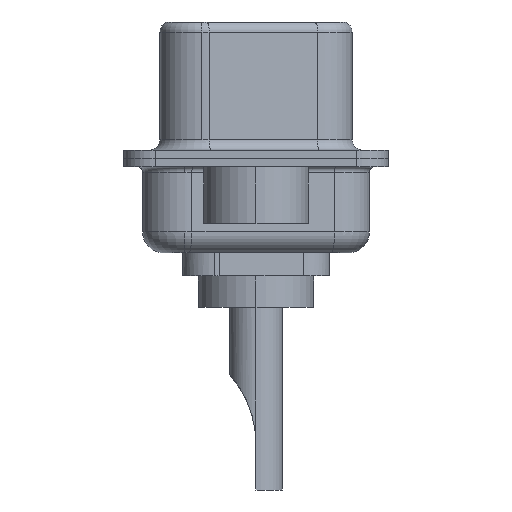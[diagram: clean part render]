
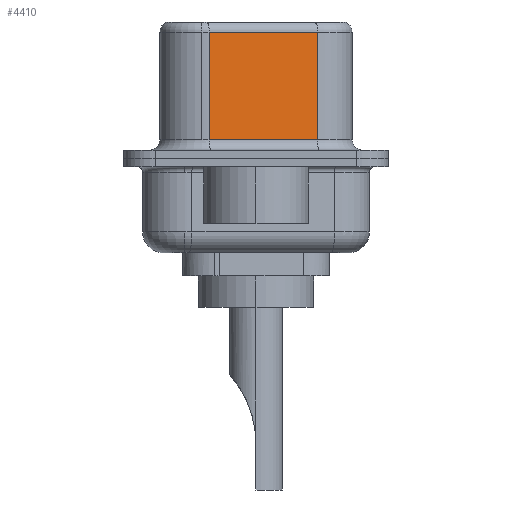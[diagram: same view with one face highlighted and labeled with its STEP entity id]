
A CAD part, left-side view. The second image highlights one B-rep face of the part: STEP entity #4410.
In plain terms, the highlighted planar face has unit normal (-0.985, -0.174, 0).
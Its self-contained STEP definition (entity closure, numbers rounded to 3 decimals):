
#92 = CARTESIAN_POINT ( 'NONE',  ( 4.585, -2.927, 6.52 ) ) ;
#216 = DIRECTION ( 'NONE',  ( 0., 0., -1. ) ) ;
#671 = VERTEX_POINT ( 'NONE', #15368 ) ;
#1027 = VERTEX_POINT ( 'NONE', #1853 ) ;
#1247 = VECTOR ( 'NONE', #216, 1000. ) ;
#1521 = DIRECTION ( 'NONE',  ( 0.174, -0.985, 0. ) ) ;
#1773 = EDGE_CURVE ( 'NONE', #671, #15665, #8259, .T. ) ;
#1853 = CARTESIAN_POINT ( 'NONE',  ( 3.675, 2.233, 6.02 ) ) ;
#1908 = FACE_OUTER_BOUND ( 'NONE', #16865, .T. ) ;
#1952 = VECTOR ( 'NONE', #1521, 1000. ) ;
#3297 = EDGE_CURVE ( 'NONE', #3618, #15665, #16054, .T. ) ;
#3618 = VERTEX_POINT ( 'NONE', #10603 ) ;
#3769 = ORIENTED_EDGE ( 'NONE', *, *, #8292, .T. ) ;
#4311 = CARTESIAN_POINT ( 'NONE',  ( 4.585, -2.927, 6.02 ) ) ;
#4410 = ADVANCED_FACE ( 'NONE', ( #1908 ), #14318, .F. ) ;
#6431 = VECTOR ( 'NONE', #6454, 1000. ) ;
#6454 = DIRECTION ( 'NONE',  ( 0., 0., -1. ) ) ;
#6577 = DIRECTION ( 'NONE',  ( -0.174, 0.985, 0. ) ) ;
#6581 = DIRECTION ( 'NONE',  ( 0.985, 0.174, 0. ) ) ;
#8259 = LINE ( 'NONE', #92, #1247 ) ;
#8292 = EDGE_CURVE ( 'NONE', #1027, #3618, #9884, .T. ) ;
#8526 = VECTOR ( 'NONE', #12195, 1000. ) ;
#9026 = CARTESIAN_POINT ( 'NONE',  ( 3.675, 2.233, 6.52 ) ) ;
#9884 = LINE ( 'NONE', #9026, #6431 ) ;
#10603 = CARTESIAN_POINT ( 'NONE',  ( 3.675, 2.233, 0.9 ) ) ;
#11206 = AXIS2_PLACEMENT_3D ( 'NONE', #13846, #6581, #6577 ) ;
#11610 = ORIENTED_EDGE ( 'NONE', *, *, #1773, .F. ) ;
#11935 = CARTESIAN_POINT ( 'NONE',  ( 4.585, -2.927, 0.9 ) ) ;
#12065 = EDGE_CURVE ( 'NONE', #671, #1027, #15632, .T. ) ;
#12195 = DIRECTION ( 'NONE',  ( -0.174, 0.985, 0. ) ) ;
#13846 = CARTESIAN_POINT ( 'NONE',  ( 4.585, -2.927, 6.52 ) ) ;
#14318 = PLANE ( 'NONE',  #11206 ) ;
#14711 = ORIENTED_EDGE ( 'NONE', *, *, #12065, .T. ) ;
#15368 = CARTESIAN_POINT ( 'NONE',  ( 4.585, -2.927, 6.02 ) ) ;
#15632 = LINE ( 'NONE', #4311, #8526 ) ;
#15665 = VERTEX_POINT ( 'NONE', #16704 ) ;
#16054 = LINE ( 'NONE', #11935, #1952 ) ;
#16704 = CARTESIAN_POINT ( 'NONE',  ( 4.585, -2.927, 0.9 ) ) ;
#16865 = EDGE_LOOP ( 'NONE', ( #11610, #14711, #3769, #17083 ) ) ;
#17083 = ORIENTED_EDGE ( 'NONE', *, *, #3297, .T. ) ;
